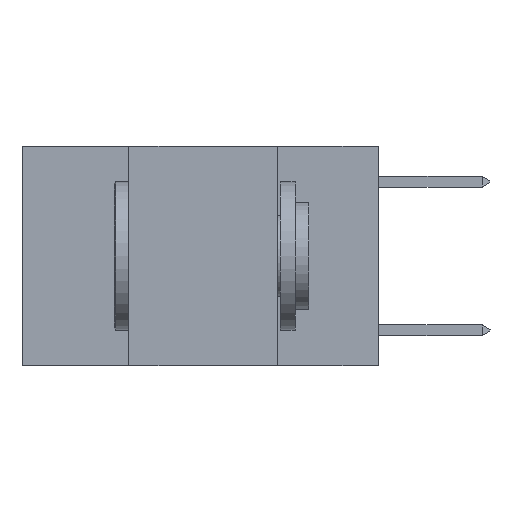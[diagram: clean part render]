
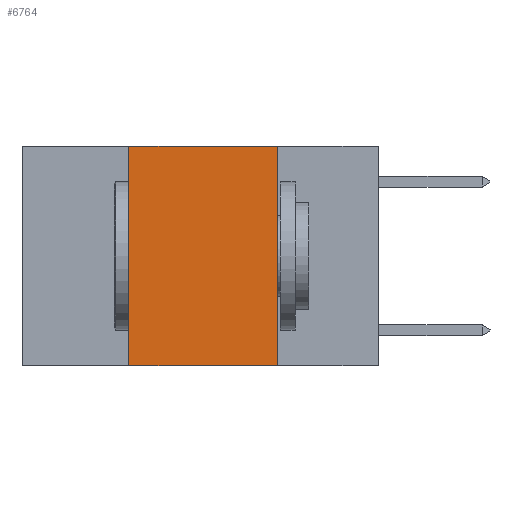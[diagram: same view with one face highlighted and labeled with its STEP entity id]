
A CAD part, left-side view. The second image highlights one B-rep face of the part: STEP entity #6764.
In plain terms, the highlighted planar face has unit normal (-1, 0, 0).
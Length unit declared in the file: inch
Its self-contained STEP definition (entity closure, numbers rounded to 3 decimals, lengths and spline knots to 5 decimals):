
#225 = CARTESIAN_POINT ( 'NONE',  ( 0., 0.17, 0. ) ) ;
#812 = LINE ( 'NONE', #6294, #7457 ) ;
#1267 = ORIENTED_EDGE ( 'NONE', *, *, #6942, .F. ) ;
#1309 = ORIENTED_EDGE ( 'NONE', *, *, #10401, .F. ) ;
#1402 = ORIENTED_EDGE ( 'NONE', *, *, #8772, .F. ) ;
#1418 = ORIENTED_EDGE ( 'NONE', *, *, #1679, .T. ) ;
#1679 = EDGE_CURVE ( 'NONE', #8743, #8730, #812, .T. ) ;
#2352 = DIRECTION ( 'NONE',  ( 0., -1., 0. ) ) ;
#2522 = CARTESIAN_POINT ( 'NONE',  ( 0., 0.17, -0.37 ) ) ;
#3341 = LINE ( 'NONE', #4545, #7007 ) ;
#3343 = CARTESIAN_POINT ( 'NONE',  ( 0., 0.42, 0. ) ) ;
#3634 = VERTEX_POINT ( 'NONE', #225 ) ;
#4194 = CARTESIAN_POINT ( 'NONE',  ( 0., 0.42, -0.37 ) ) ;
#4364 = CARTESIAN_POINT ( 'NONE',  ( 0., 0.6, 0. ) ) ;
#4545 = CARTESIAN_POINT ( 'NONE',  ( 0., 0.17, 0. ) ) ;
#5004 = VECTOR ( 'NONE', #2352, 39.37008 ) ;
#5235 = DIRECTION ( 'NONE',  ( 0., 0., -1. ) ) ;
#6294 = CARTESIAN_POINT ( 'NONE',  ( 0., 0.6, -0.37 ) ) ;
#6381 = FACE_OUTER_BOUND ( 'NONE', #7628, .T. ) ;
#6533 = DIRECTION ( 'NONE',  ( 0., -1., 0. ) ) ;
#6764 = ADVANCED_FACE ( 'NONE', ( #6381 ), #7668, .F. ) ;
#6942 = EDGE_CURVE ( 'NONE', #3634, #8730, #3341, .T. ) ;
#6977 = VECTOR ( 'NONE', #9887, 39.37008 ) ;
#7007 = VECTOR ( 'NONE', #7043, 39.37008 ) ;
#7019 = VERTEX_POINT ( 'NONE', #7076 ) ;
#7043 = DIRECTION ( 'NONE',  ( 0., 0., -1. ) ) ;
#7076 = CARTESIAN_POINT ( 'NONE',  ( 0., 0.42, 0. ) ) ;
#7457 = VECTOR ( 'NONE', #6533, 39.37008 ) ;
#7628 = EDGE_LOOP ( 'NONE', ( #1267, #1309, #1402, #1418 ) ) ;
#7668 = PLANE ( 'NONE',  #10008 ) ;
#8123 = CARTESIAN_POINT ( 'NONE',  ( 0., 0.6, 0. ) ) ;
#8591 = LINE ( 'NONE', #3343, #6977 ) ;
#8730 = VERTEX_POINT ( 'NONE', #2522 ) ;
#8743 = VERTEX_POINT ( 'NONE', #4194 ) ;
#8772 = EDGE_CURVE ( 'NONE', #8743, #7019, #8591, .T. ) ;
#9057 = LINE ( 'NONE', #8123, #5004 ) ;
#9887 = DIRECTION ( 'NONE',  ( 0., 0., 1. ) ) ;
#9994 = DIRECTION ( 'NONE',  ( 1., 0., 0. ) ) ;
#10008 = AXIS2_PLACEMENT_3D ( 'NONE', #4364, #9994, #5235 ) ;
#10401 = EDGE_CURVE ( 'NONE', #7019, #3634, #9057, .T. ) ;
